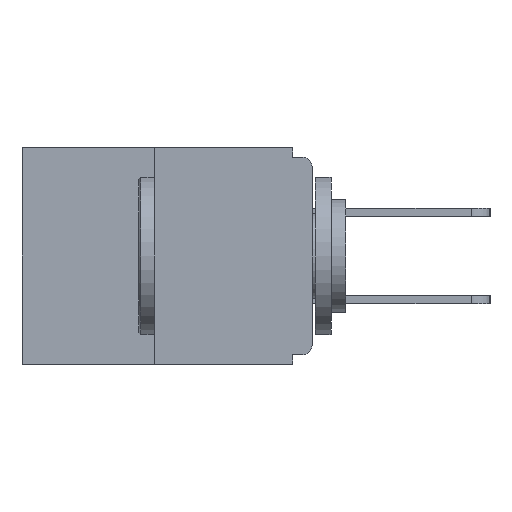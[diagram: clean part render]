
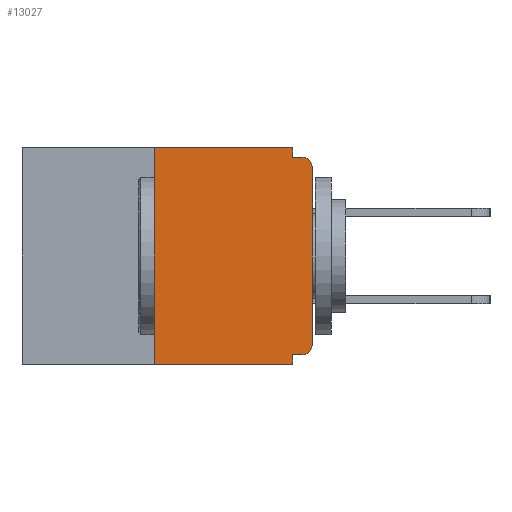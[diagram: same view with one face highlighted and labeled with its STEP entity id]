
A CAD part, left-side view. The second image highlights one B-rep face of the part: STEP entity #13027.
In plain terms, the highlighted planar face has unit normal (-1, 0, 0).
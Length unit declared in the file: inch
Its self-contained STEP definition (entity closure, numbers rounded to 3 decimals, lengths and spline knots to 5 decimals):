
#471 = LINE ( 'NONE', #7149, #19955 ) ;
#1197 = AXIS2_PLACEMENT_3D ( 'NONE', #9069, #9325, #24275 ) ;
#1330 = CARTESIAN_POINT ( 'NONE',  ( 0., 0., 0. ) ) ;
#1343 = EDGE_CURVE ( 'NONE', #2903, #11924, #22145, .T. ) ;
#1906 = CARTESIAN_POINT ( 'NONE',  ( 0., 0.46, 0. ) ) ;
#1961 = EDGE_CURVE ( 'NONE', #8584, #9984, #16783, .T. ) ;
#2322 = ORIENTED_EDGE ( 'NONE', *, *, #3088, .T. ) ;
#2903 = VERTEX_POINT ( 'NONE', #13712 ) ;
#2935 = VECTOR ( 'NONE', #12918, 39.37008 ) ;
#2937 = CARTESIAN_POINT ( 'NONE',  ( 0., 0.015, -0.03 ) ) ;
#3088 = EDGE_CURVE ( 'NONE', #24085, #2903, #4945, .T. ) ;
#3579 = CARTESIAN_POINT ( 'NONE',  ( 0., 0., -0.313 ) ) ;
#3771 = DIRECTION ( 'NONE',  ( 0., 0., -1. ) ) ;
#3895 = ORIENTED_EDGE ( 'NONE', *, *, #17186, .T. ) ;
#3947 = CARTESIAN_POINT ( 'NONE',  ( 0., 0.031, 0. ) ) ;
#4002 = LINE ( 'NONE', #16661, #14599 ) ;
#4008 = DIRECTION ( 'NONE',  ( 0., -1., 0. ) ) ;
#4219 = CARTESIAN_POINT ( 'NONE',  ( 0., 0., -0.328 ) ) ;
#4945 = LINE ( 'NONE', #1330, #24423 ) ;
#5232 = LINE ( 'NONE', #15257, #17301 ) ;
#5381 = DIRECTION ( 'NONE',  ( 0., -1., 0. ) ) ;
#5463 = CARTESIAN_POINT ( 'NONE',  ( 0., 0.015, -0.015 ) ) ;
#5857 = DIRECTION ( 'NONE',  ( 0., 1., 0. ) ) ;
#7052 = VERTEX_POINT ( 'NONE', #19170 ) ;
#7149 = CARTESIAN_POINT ( 'NONE',  ( 0., 0.46, -0.343 ) ) ;
#7791 = ORIENTED_EDGE ( 'NONE', *, *, #1961, .F. ) ;
#7905 = CIRCLE ( 'NONE', #1197, 0.015 ) ;
#8040 = FACE_OUTER_BOUND ( 'NONE', #10685, .T. ) ;
#8221 = ORIENTED_EDGE ( 'NONE', *, *, #23560, .F. ) ;
#8451 = VERTEX_POINT ( 'NONE', #15633 ) ;
#8584 = VERTEX_POINT ( 'NONE', #22000 ) ;
#9069 = CARTESIAN_POINT ( 'NONE',  ( 0., 0.015, -0.313 ) ) ;
#9079 = DIRECTION ( 'NONE',  ( 1., 0., 0. ) ) ;
#9127 = ORIENTED_EDGE ( 'NONE', *, *, #1343, .T. ) ;
#9325 = DIRECTION ( 'NONE',  ( -1., 0., 0. ) ) ;
#9984 = VERTEX_POINT ( 'NONE', #11158 ) ;
#10106 = EDGE_CURVE ( 'NONE', #14504, #11924, #5232, .T. ) ;
#10459 = LINE ( 'NONE', #3947, #22624 ) ;
#10685 = EDGE_LOOP ( 'NONE', ( #13925, #8221, #3895, #7791, #16522, #23439, #2322, #9127, #24461, #17197 ) ) ;
#10866 = CARTESIAN_POINT ( 'NONE',  ( 0., 0.031, -0.343 ) ) ;
#11158 = CARTESIAN_POINT ( 'NONE',  ( 0., 0.031, -0.343 ) ) ;
#11240 = DIRECTION ( 'NONE',  ( 0., 0., -1. ) ) ;
#11549 = EDGE_CURVE ( 'NONE', #7052, #14504, #10459, .T. ) ;
#11924 = VERTEX_POINT ( 'NONE', #5463 ) ;
#12047 = EDGE_CURVE ( 'NONE', #14265, #7052, #4002, .T. ) ;
#12918 = DIRECTION ( 'NONE',  ( 0., 0., -1. ) ) ;
#13027 = ADVANCED_FACE ( 'NONE', ( #8040 ), #13036, .F. ) ;
#13036 = PLANE ( 'NONE',  #21198 ) ;
#13648 = CARTESIAN_POINT ( 'NONE',  ( 0., 0.031, -0.015 ) ) ;
#13712 = CARTESIAN_POINT ( 'NONE',  ( 0., 0., -0.03 ) ) ;
#13925 = ORIENTED_EDGE ( 'NONE', *, *, #12047, .F. ) ;
#14265 = VERTEX_POINT ( 'NONE', #15116 ) ;
#14504 = VERTEX_POINT ( 'NONE', #13648 ) ;
#14599 = VECTOR ( 'NONE', #5381, 39.37008 ) ;
#15112 = CARTESIAN_POINT ( 'NONE',  ( 0., 0.25, 0. ) ) ;
#15116 = CARTESIAN_POINT ( 'NONE',  ( 0., 0.25, 0. ) ) ;
#15257 = CARTESIAN_POINT ( 'NONE',  ( 0., 0., -0.015 ) ) ;
#15517 = EDGE_CURVE ( 'NONE', #23047, #24085, #7905, .T. ) ;
#15633 = CARTESIAN_POINT ( 'NONE',  ( 0., 0.25, -0.343 ) ) ;
#16522 = ORIENTED_EDGE ( 'NONE', *, *, #22375, .F. ) ;
#16661 = CARTESIAN_POINT ( 'NONE',  ( 0., 0.46, 0. ) ) ;
#16783 = LINE ( 'NONE', #10866, #2935 ) ;
#17186 = EDGE_CURVE ( 'NONE', #8451, #9984, #471, .T. ) ;
#17197 = ORIENTED_EDGE ( 'NONE', *, *, #11549, .F. ) ;
#17301 = VECTOR ( 'NONE', #4008, 39.37008 ) ;
#17907 = DIRECTION ( 'NONE',  ( -1., 0., 0. ) ) ;
#18680 = VECTOR ( 'NONE', #21044, 39.37008 ) ;
#19170 = CARTESIAN_POINT ( 'NONE',  ( 0., 0.031, 0. ) ) ;
#19231 = CARTESIAN_POINT ( 'NONE',  ( 0., 0.015, -0.328 ) ) ;
#19955 = VECTOR ( 'NONE', #22173, 39.37008 ) ;
#20225 = AXIS2_PLACEMENT_3D ( 'NONE', #2937, #17907, #21725 ) ;
#20290 = DIRECTION ( 'NONE',  ( 0., 0., 1. ) ) ;
#21044 = DIRECTION ( 'NONE',  ( 0., 0., 1. ) ) ;
#21198 = AXIS2_PLACEMENT_3D ( 'NONE', #1906, #9079, #11240 ) ;
#21725 = DIRECTION ( 'NONE',  ( 0., 0., -1. ) ) ;
#22000 = CARTESIAN_POINT ( 'NONE',  ( 0., 0.031, -0.328 ) ) ;
#22145 = CIRCLE ( 'NONE', #20225, 0.015 ) ;
#22173 = DIRECTION ( 'NONE',  ( 0., -1., 0. ) ) ;
#22375 = EDGE_CURVE ( 'NONE', #23047, #8584, #22944, .T. ) ;
#22580 = LINE ( 'NONE', #15112, #18680 ) ;
#22624 = VECTOR ( 'NONE', #3771, 39.37008 ) ;
#22944 = LINE ( 'NONE', #4219, #23535 ) ;
#23047 = VERTEX_POINT ( 'NONE', #19231 ) ;
#23439 = ORIENTED_EDGE ( 'NONE', *, *, #15517, .T. ) ;
#23535 = VECTOR ( 'NONE', #5857, 39.37008 ) ;
#23560 = EDGE_CURVE ( 'NONE', #8451, #14265, #22580, .T. ) ;
#24085 = VERTEX_POINT ( 'NONE', #3579 ) ;
#24275 = DIRECTION ( 'NONE',  ( 0., 0., -1. ) ) ;
#24423 = VECTOR ( 'NONE', #20290, 39.37008 ) ;
#24461 = ORIENTED_EDGE ( 'NONE', *, *, #10106, .F. ) ;
